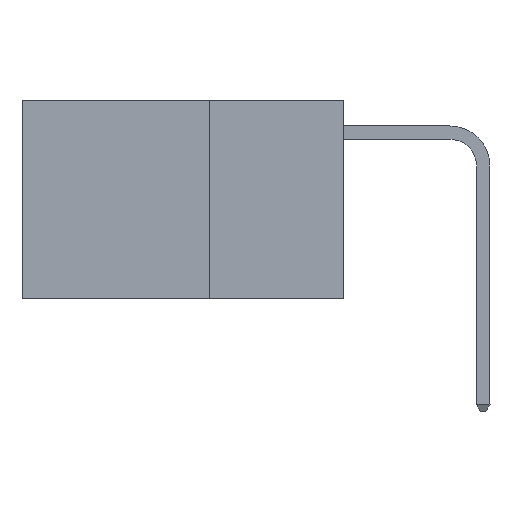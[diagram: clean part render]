
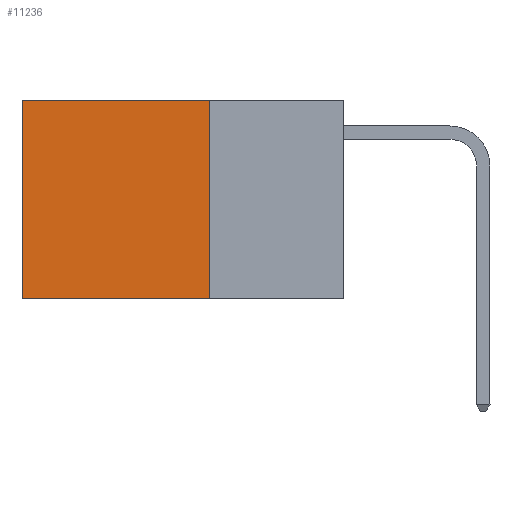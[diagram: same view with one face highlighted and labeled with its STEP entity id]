
A CAD part, left-side view. The second image highlights one B-rep face of the part: STEP entity #11236.
In plain terms, the highlighted planar face has unit normal (-1, 0, 0).
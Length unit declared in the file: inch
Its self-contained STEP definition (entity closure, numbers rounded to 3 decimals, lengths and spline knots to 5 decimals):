
#346 = CARTESIAN_POINT ( 'NONE',  ( 0.2625, 0.25, 0. ) ) ;
#2427 = ORIENTED_EDGE ( 'NONE', *, *, #19024, .T. ) ;
#2776 = VECTOR ( 'NONE', #17096, 39.37008 ) ;
#2826 = LINE ( 'NONE', #6813, #2776 ) ;
#3939 = VERTEX_POINT ( 'NONE', #18342 ) ;
#4129 = LINE ( 'NONE', #13711, #19778 ) ;
#4708 = CARTESIAN_POINT ( 'NONE',  ( 0.2625, 0.6, 0. ) ) ;
#5070 = VERTEX_POINT ( 'NONE', #14827 ) ;
#6147 = DIRECTION ( 'NONE',  ( 0., 0., -1. ) ) ;
#6293 = DIRECTION ( 'NONE',  ( 0., 0., -1. ) ) ;
#6404 = CARTESIAN_POINT ( 'NONE',  ( 0.2625, 0.25, 0. ) ) ;
#6813 = CARTESIAN_POINT ( 'NONE',  ( 0.2625, 0.25, -0.37 ) ) ;
#7322 = ORIENTED_EDGE ( 'NONE', *, *, #8441, .F. ) ;
#7466 = VECTOR ( 'NONE', #6293, 39.37008 ) ;
#7843 = DIRECTION ( 'NONE',  ( 1., 0., 0. ) ) ;
#8288 = LINE ( 'NONE', #11076, #15936 ) ;
#8441 = EDGE_CURVE ( 'NONE', #14320, #3939, #2826, .T. ) ;
#10425 = PLANE ( 'NONE',  #12534 ) ;
#11076 = CARTESIAN_POINT ( 'NONE',  ( 0.2625, 0.25, 0. ) ) ;
#11178 = ORIENTED_EDGE ( 'NONE', *, *, #13708, .T. ) ;
#11236 = ADVANCED_FACE ( 'NONE', ( #16955 ), #10425, .F. ) ;
#12534 = AXIS2_PLACEMENT_3D ( 'NONE', #346, #7843, #6147 ) ;
#12609 = DIRECTION ( 'NONE',  ( 0., 0., -1. ) ) ;
#12904 = ORIENTED_EDGE ( 'NONE', *, *, #16540, .F. ) ;
#12944 = DIRECTION ( 'NONE',  ( 0., 1., 0. ) ) ;
#13708 = EDGE_CURVE ( 'NONE', #15897, #5070, #4129, .T. ) ;
#13711 = CARTESIAN_POINT ( 'NONE',  ( 0.2625, 0.25, 0. ) ) ;
#14320 = VERTEX_POINT ( 'NONE', #18727 ) ;
#14827 = CARTESIAN_POINT ( 'NONE',  ( 0.2625, 0.6, 0. ) ) ;
#15637 = LINE ( 'NONE', #4708, #7466 ) ;
#15897 = VERTEX_POINT ( 'NONE', #6404 ) ;
#15936 = VECTOR ( 'NONE', #12609, 39.37008 ) ;
#16540 = EDGE_CURVE ( 'NONE', #15897, #14320, #8288, .T. ) ;
#16955 = FACE_OUTER_BOUND ( 'NONE', #17147, .T. ) ;
#17096 = DIRECTION ( 'NONE',  ( 0., 1., 0. ) ) ;
#17147 = EDGE_LOOP ( 'NONE', ( #2427, #7322, #12904, #11178 ) ) ;
#18342 = CARTESIAN_POINT ( 'NONE',  ( 0.2625, 0.6, -0.37 ) ) ;
#18727 = CARTESIAN_POINT ( 'NONE',  ( 0.2625, 0.25, -0.37 ) ) ;
#19024 = EDGE_CURVE ( 'NONE', #5070, #3939, #15637, .T. ) ;
#19778 = VECTOR ( 'NONE', #12944, 39.37008 ) ;
